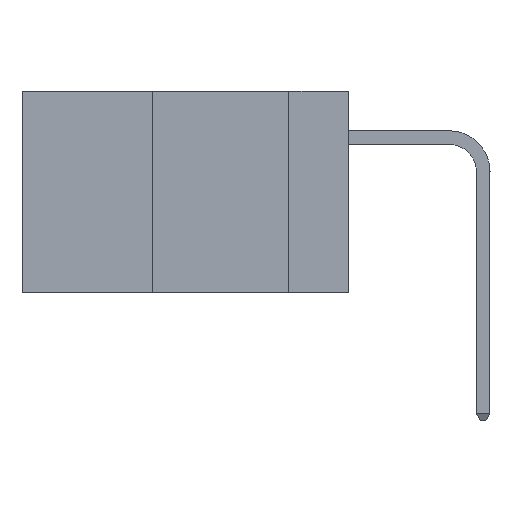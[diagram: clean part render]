
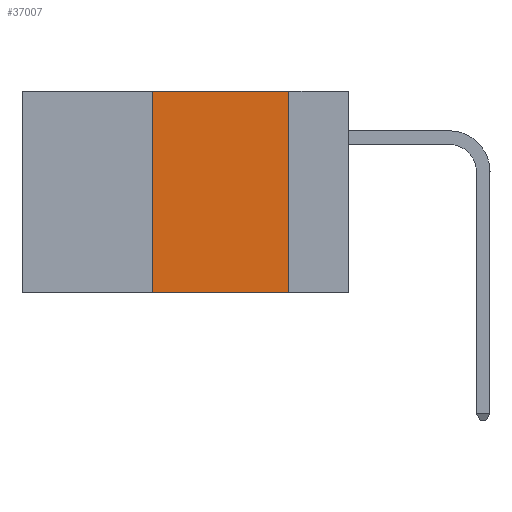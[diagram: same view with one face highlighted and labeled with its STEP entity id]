
A CAD part, left-side view. The second image highlights one B-rep face of the part: STEP entity #37007.
In plain terms, the highlighted planar face has unit normal (-1, 0, 0).
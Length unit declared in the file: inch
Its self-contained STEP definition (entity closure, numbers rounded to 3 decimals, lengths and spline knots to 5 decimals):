
#966 = AXIS2_PLACEMENT_3D ( 'NONE', #27438, #10178, #30305 ) ;
#1817 = LINE ( 'NONE', #28333, #23990 ) ;
#3493 = CARTESIAN_POINT ( 'NONE',  ( 0., 0.36, 0. ) ) ;
#3691 = VERTEX_POINT ( 'NONE', #25012 ) ;
#3971 = VECTOR ( 'NONE', #10600, 39.37008 ) ;
#6081 = CARTESIAN_POINT ( 'NONE',  ( 0., 0.11, 0. ) ) ;
#7283 = VECTOR ( 'NONE', #9322, 39.37008 ) ;
#7707 = CARTESIAN_POINT ( 'NONE',  ( 0., 0.6, 0. ) ) ;
#9322 = DIRECTION ( 'NONE',  ( 0., 0., 1. ) ) ;
#10178 = DIRECTION ( 'NONE',  ( 1., 0., 0. ) ) ;
#10600 = DIRECTION ( 'NONE',  ( 0., -1., 0. ) ) ;
#10722 = VERTEX_POINT ( 'NONE', #35836 ) ;
#12372 = EDGE_LOOP ( 'NONE', ( #15828, #13151, #36154, #30825 ) ) ;
#12580 = CARTESIAN_POINT ( 'NONE',  ( 0., 0.11, -0.37 ) ) ;
#12765 = EDGE_CURVE ( 'NONE', #30430, #30092, #1817, .T. ) ;
#13151 = ORIENTED_EDGE ( 'NONE', *, *, #27880, .F. ) ;
#13330 = FACE_OUTER_BOUND ( 'NONE', #12372, .T. ) ;
#15435 = LINE ( 'NONE', #6081, #29853 ) ;
#15828 = ORIENTED_EDGE ( 'NONE', *, *, #25622, .F. ) ;
#17661 = DIRECTION ( 'NONE',  ( 0., 0., -1. ) ) ;
#19339 = LINE ( 'NONE', #7707, #3971 ) ;
#22649 = LINE ( 'NONE', #3493, #7283 ) ;
#23990 = VECTOR ( 'NONE', #31222, 39.37008 ) ;
#25012 = CARTESIAN_POINT ( 'NONE',  ( 0., 0.11, 0. ) ) ;
#25622 = EDGE_CURVE ( 'NONE', #3691, #30092, #15435, .T. ) ;
#26314 = EDGE_CURVE ( 'NONE', #30430, #10722, #22649, .T. ) ;
#27438 = CARTESIAN_POINT ( 'NONE',  ( 0., 0.6, 0. ) ) ;
#27880 = EDGE_CURVE ( 'NONE', #10722, #3691, #19339, .T. ) ;
#28333 = CARTESIAN_POINT ( 'NONE',  ( 0., 0.6, -0.37 ) ) ;
#29853 = VECTOR ( 'NONE', #17661, 39.37008 ) ;
#30092 = VERTEX_POINT ( 'NONE', #12580 ) ;
#30305 = DIRECTION ( 'NONE',  ( 0., 0., -1. ) ) ;
#30430 = VERTEX_POINT ( 'NONE', #31447 ) ;
#30825 = ORIENTED_EDGE ( 'NONE', *, *, #12765, .T. ) ;
#31222 = DIRECTION ( 'NONE',  ( 0., -1., 0. ) ) ;
#31447 = CARTESIAN_POINT ( 'NONE',  ( 0., 0.36, -0.37 ) ) ;
#35836 = CARTESIAN_POINT ( 'NONE',  ( 0., 0.36, 0. ) ) ;
#35921 = PLANE ( 'NONE',  #966 ) ;
#36154 = ORIENTED_EDGE ( 'NONE', *, *, #26314, .F. ) ;
#37007 = ADVANCED_FACE ( 'NONE', ( #13330 ), #35921, .F. ) ;
